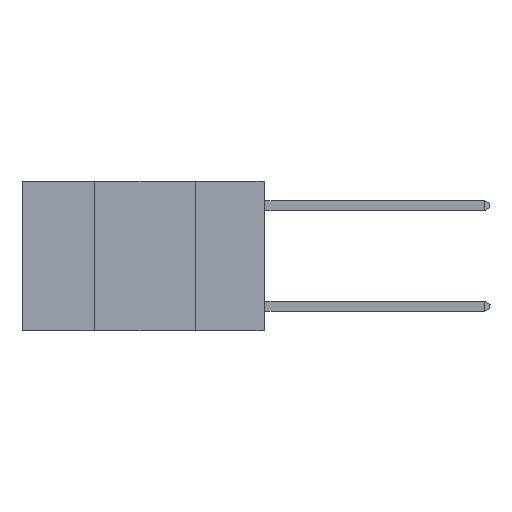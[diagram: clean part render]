
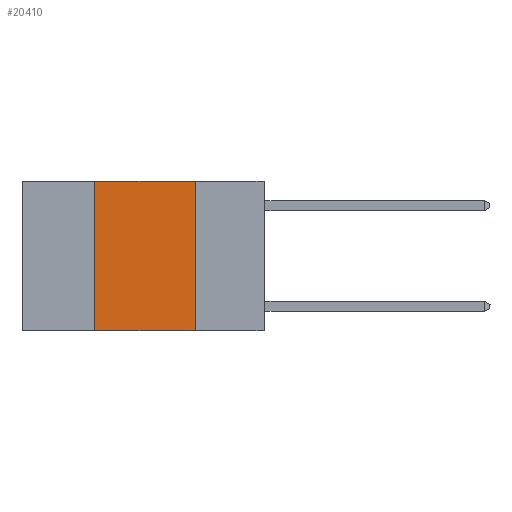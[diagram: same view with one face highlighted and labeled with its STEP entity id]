
A CAD part, left-side view. The second image highlights one B-rep face of the part: STEP entity #20410.
In plain terms, the highlighted planar face has unit normal (-1, 0, 0).
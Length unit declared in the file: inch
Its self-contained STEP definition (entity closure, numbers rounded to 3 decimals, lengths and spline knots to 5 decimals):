
#347 = ORIENTED_EDGE ( 'NONE', *, *, #1486, .F. ) ;
#1486 = EDGE_CURVE ( 'NONE', #4079, #11222, #9251, .T. ) ;
#2022 = DIRECTION ( 'NONE',  ( 1., 0., 0. ) ) ;
#2965 = CARTESIAN_POINT ( 'NONE',  ( 0., 0.42, -0.37 ) ) ;
#3184 = EDGE_CURVE ( 'NONE', #12019, #4079, #19659, .T. ) ;
#4079 = VERTEX_POINT ( 'NONE', #6731 ) ;
#4503 = VECTOR ( 'NONE', #4700, 39.37008 ) ;
#4700 = DIRECTION ( 'NONE',  ( 0., -1., 0. ) ) ;
#5934 = CARTESIAN_POINT ( 'NONE',  ( 0., 0.6, -0.37 ) ) ;
#5956 = LINE ( 'NONE', #6434, #10067 ) ;
#6026 = ORIENTED_EDGE ( 'NONE', *, *, #6946, .T. ) ;
#6434 = CARTESIAN_POINT ( 'NONE',  ( 0., 0.17, 0. ) ) ;
#6710 = DIRECTION ( 'NONE',  ( 0., 0., 1. ) ) ;
#6731 = CARTESIAN_POINT ( 'NONE',  ( 0., 0.42, 0. ) ) ;
#6946 = EDGE_CURVE ( 'NONE', #12019, #8129, #21693, .T. ) ;
#7725 = DIRECTION ( 'NONE',  ( 0., -1., 0. ) ) ;
#7742 = EDGE_LOOP ( 'NONE', ( #14213, #347, #19324, #6026 ) ) ;
#8129 = VERTEX_POINT ( 'NONE', #12122 ) ;
#9251 = LINE ( 'NONE', #20355, #4503 ) ;
#10067 = VECTOR ( 'NONE', #21953, 39.37008 ) ;
#10483 = VECTOR ( 'NONE', #6710, 39.37008 ) ;
#11222 = VERTEX_POINT ( 'NONE', #22203 ) ;
#11765 = FACE_OUTER_BOUND ( 'NONE', #7742, .T. ) ;
#12019 = VERTEX_POINT ( 'NONE', #2965 ) ;
#12122 = CARTESIAN_POINT ( 'NONE',  ( 0., 0.17, -0.37 ) ) ;
#12783 = CARTESIAN_POINT ( 'NONE',  ( 0., 0.6, 0. ) ) ;
#14213 = ORIENTED_EDGE ( 'NONE', *, *, #16251, .F. ) ;
#14540 = DIRECTION ( 'NONE',  ( 0., 0., -1. ) ) ;
#15379 = CARTESIAN_POINT ( 'NONE',  ( 0., 0.42, 0. ) ) ;
#16251 = EDGE_CURVE ( 'NONE', #11222, #8129, #5956, .T. ) ;
#17206 = VECTOR ( 'NONE', #7725, 39.37008 ) ;
#17824 = AXIS2_PLACEMENT_3D ( 'NONE', #12783, #2022, #14540 ) ;
#19324 = ORIENTED_EDGE ( 'NONE', *, *, #3184, .F. ) ;
#19629 = PLANE ( 'NONE',  #17824 ) ;
#19659 = LINE ( 'NONE', #15379, #10483 ) ;
#20355 = CARTESIAN_POINT ( 'NONE',  ( 0., 0.6, 0. ) ) ;
#20410 = ADVANCED_FACE ( 'NONE', ( #11765 ), #19629, .F. ) ;
#21693 = LINE ( 'NONE', #5934, #17206 ) ;
#21953 = DIRECTION ( 'NONE',  ( 0., 0., -1. ) ) ;
#22203 = CARTESIAN_POINT ( 'NONE',  ( 0., 0.17, 0. ) ) ;
